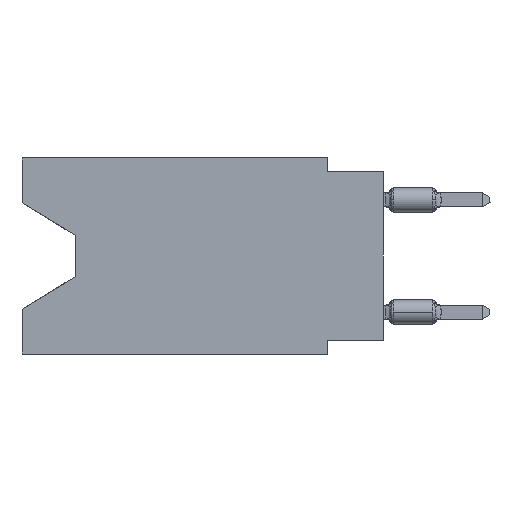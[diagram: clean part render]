
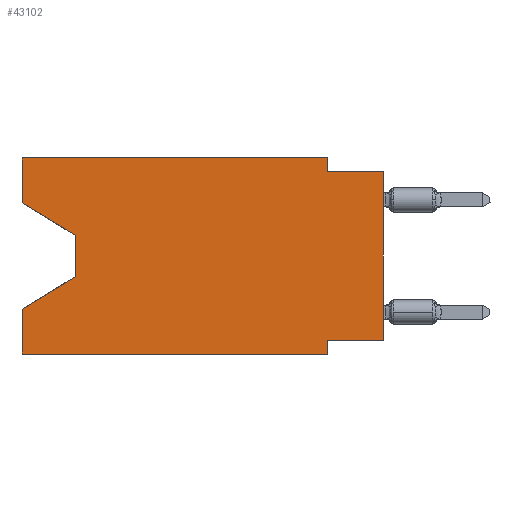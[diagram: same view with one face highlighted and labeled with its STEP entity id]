
A CAD part, left-side view. The second image highlights one B-rep face of the part: STEP entity #43102.
In plain terms, the highlighted planar face has unit normal (-1, 0, 0).
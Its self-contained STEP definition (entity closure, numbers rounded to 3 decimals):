
#617 = LINE ( 'NONE', #54633, #27802 ) ;
#1306 = VERTEX_POINT ( 'NONE', #27638 ) ;
#1836 = DIRECTION ( 'NONE',  ( 0., -1., 0. ) ) ;
#2307 = VERTEX_POINT ( 'NONE', #68463 ) ;
#2730 = EDGE_CURVE ( 'NONE', #19771, #59500, #4900, .T. ) ;
#3087 = DIRECTION ( 'NONE',  ( 0., 1., 0. ) ) ;
#3931 = DIRECTION ( 'NONE',  ( 0., -1., 0. ) ) ;
#4218 = ORIENTED_EDGE ( 'NONE', *, *, #52696, .F. ) ;
#4465 = LINE ( 'NONE', #56448, #4756 ) ;
#4756 = VECTOR ( 'NONE', #3087, 1000. ) ;
#4897 = VECTOR ( 'NONE', #27352, 1000. ) ;
#4900 = LINE ( 'NONE', #68368, #45089 ) ;
#5385 = CARTESIAN_POINT ( 'NONE',  ( 0., 16.383, 0. ) ) ;
#5423 = LINE ( 'NONE', #26704, #20906 ) ;
#5783 = EDGE_CURVE ( 'NONE', #59500, #37908, #5423, .T. ) ;
#5933 = VECTOR ( 'NONE', #34104, 1000. ) ;
#8051 = ORIENTED_EDGE ( 'NONE', *, *, #11867, .F. ) ;
#8557 = VECTOR ( 'NONE', #19544, 1000. ) ;
#9963 = DIRECTION ( 'NONE',  ( 0., 0.855, -0.519 ) ) ;
#11725 = ORIENTED_EDGE ( 'NONE', *, *, #42154, .T. ) ;
#11867 = EDGE_CURVE ( 'NONE', #49075, #37908, #66022, .T. ) ;
#11931 = CARTESIAN_POINT ( 'NONE',  ( 0., 2.54, -8.89 ) ) ;
#13270 = ORIENTED_EDGE ( 'NONE', *, *, #65249, .T. ) ;
#13945 = PLANE ( 'NONE',  #50484 ) ;
#14165 = VERTEX_POINT ( 'NONE', #53018 ) ;
#14279 = DIRECTION ( 'NONE',  ( 0., 0., -1. ) ) ;
#14666 = LINE ( 'NONE', #20944, #49072 ) ;
#15368 = LINE ( 'NONE', #58949, #54455 ) ;
#15716 = DIRECTION ( 'NONE',  ( 0., -1., 0. ) ) ;
#15976 = EDGE_CURVE ( 'NONE', #1306, #50974, #45350, .T. ) ;
#16616 = ORIENTED_EDGE ( 'NONE', *, *, #5783, .T. ) ;
#17039 = ORIENTED_EDGE ( 'NONE', *, *, #15976, .F. ) ;
#19544 = DIRECTION ( 'NONE',  ( 0., 0., -1. ) ) ;
#19771 = VERTEX_POINT ( 'NONE', #51970 ) ;
#19848 = EDGE_CURVE ( 'NONE', #2307, #37178, #14666, .T. ) ;
#20010 = CARTESIAN_POINT ( 'NONE',  ( 0., 16.383, 0. ) ) ;
#20029 = CARTESIAN_POINT ( 'NONE',  ( 0., 16.383, -2.038 ) ) ;
#20906 = VECTOR ( 'NONE', #9963, 1000. ) ;
#20944 = CARTESIAN_POINT ( 'NONE',  ( 0., 0., 0. ) ) ;
#21397 = EDGE_CURVE ( 'NONE', #14165, #37178, #51700, .T. ) ;
#23742 = CARTESIAN_POINT ( 'NONE',  ( 0., 2.54, -8.89 ) ) ;
#24390 = CARTESIAN_POINT ( 'NONE',  ( 0., 16.383, 0. ) ) ;
#26704 = CARTESIAN_POINT ( 'NONE',  ( 0., 13.97, -5.385 ) ) ;
#26950 = EDGE_CURVE ( 'NONE', #49923, #14165, #617, .T. ) ;
#27352 = DIRECTION ( 'NONE',  ( 0., 0., 1. ) ) ;
#27638 = CARTESIAN_POINT ( 'NONE',  ( 0., 2.54, -8.255 ) ) ;
#27802 = VECTOR ( 'NONE', #38603, 1000. ) ;
#28350 = CARTESIAN_POINT ( 'NONE',  ( 0., 16.383, -8.89 ) ) ;
#29972 = FACE_OUTER_BOUND ( 'NONE', #57995, .T. ) ;
#34005 = ORIENTED_EDGE ( 'NONE', *, *, #19848, .T. ) ;
#34104 = DIRECTION ( 'NONE',  ( 0., -0.855, -0.519 ) ) ;
#34168 = VERTEX_POINT ( 'NONE', #53078 ) ;
#34519 = DIRECTION ( 'NONE',  ( 1., 0., 0. ) ) ;
#34909 = CARTESIAN_POINT ( 'NONE',  ( 0., 2.54, 0. ) ) ;
#35396 = CARTESIAN_POINT ( 'NONE',  ( 0., 16.383, -8.89 ) ) ;
#36619 = CARTESIAN_POINT ( 'NONE',  ( 0., 13.97, -5.385 ) ) ;
#36625 = DIRECTION ( 'NONE',  ( 0., 0., -1. ) ) ;
#37178 = VERTEX_POINT ( 'NONE', #68458 ) ;
#37908 = VERTEX_POINT ( 'NONE', #45283 ) ;
#38603 = DIRECTION ( 'NONE',  ( 0., 0., -1. ) ) ;
#39521 = DIRECTION ( 'NONE',  ( 0., 0., 1. ) ) ;
#39584 = VERTEX_POINT ( 'NONE', #20010 ) ;
#41589 = CARTESIAN_POINT ( 'NONE',  ( 0., 0., -0.635 ) ) ;
#42009 = ORIENTED_EDGE ( 'NONE', *, *, #2730, .T. ) ;
#42154 = EDGE_CURVE ( 'NONE', #49075, #50974, #54835, .T. ) ;
#43102 = ADVANCED_FACE ( 'NONE', ( #29972 ), #13945, .F. ) ;
#43617 = EDGE_CURVE ( 'NONE', #34168, #39584, #53839, .T. ) ;
#43646 = VECTOR ( 'NONE', #39521, 1000. ) ;
#45089 = VECTOR ( 'NONE', #36625, 1000. ) ;
#45283 = CARTESIAN_POINT ( 'NONE',  ( 0., 16.383, -6.852 ) ) ;
#45350 = LINE ( 'NONE', #23742, #8557 ) ;
#45729 = ORIENTED_EDGE ( 'NONE', *, *, #66493, .F. ) ;
#48382 = CARTESIAN_POINT ( 'NONE',  ( 0., 16.383, 0. ) ) ;
#49072 = VECTOR ( 'NONE', #58599, 1000. ) ;
#49075 = VERTEX_POINT ( 'NONE', #35396 ) ;
#49923 = VERTEX_POINT ( 'NONE', #34909 ) ;
#50484 = AXIS2_PLACEMENT_3D ( 'NONE', #24390, #34519, #14279 ) ;
#50974 = VERTEX_POINT ( 'NONE', #11931 ) ;
#51513 = VECTOR ( 'NONE', #1836, 1000. ) ;
#51700 = LINE ( 'NONE', #41589, #63679 ) ;
#51970 = CARTESIAN_POINT ( 'NONE',  ( 0., 13.97, -3.505 ) ) ;
#52696 = EDGE_CURVE ( 'NONE', #2307, #1306, #4465, .T. ) ;
#53018 = CARTESIAN_POINT ( 'NONE',  ( 0., 2.54, -0.635 ) ) ;
#53078 = CARTESIAN_POINT ( 'NONE',  ( 0., 16.383, -2.038 ) ) ;
#53839 = LINE ( 'NONE', #5385, #4897 ) ;
#54455 = VECTOR ( 'NONE', #15716, 1000. ) ;
#54633 = CARTESIAN_POINT ( 'NONE',  ( 0., 2.54, 0. ) ) ;
#54835 = LINE ( 'NONE', #28350, #51513 ) ;
#56448 = CARTESIAN_POINT ( 'NONE',  ( 0., 0., -8.255 ) ) ;
#56814 = ORIENTED_EDGE ( 'NONE', *, *, #21397, .F. ) ;
#57431 = ORIENTED_EDGE ( 'NONE', *, *, #43617, .F. ) ;
#57995 = EDGE_LOOP ( 'NONE', ( #13270, #42009, #16616, #8051, #11725, #17039, #4218, #34005, #56814, #58733, #45729, #57431 ) ) ;
#58599 = DIRECTION ( 'NONE',  ( 0., 0., 1. ) ) ;
#58733 = ORIENTED_EDGE ( 'NONE', *, *, #26950, .F. ) ;
#58949 = CARTESIAN_POINT ( 'NONE',  ( 0., 16.383, 0. ) ) ;
#59500 = VERTEX_POINT ( 'NONE', #36619 ) ;
#63679 = VECTOR ( 'NONE', #3931, 1000. ) ;
#65249 = EDGE_CURVE ( 'NONE', #34168, #19771, #67800, .T. ) ;
#66022 = LINE ( 'NONE', #48382, #43646 ) ;
#66493 = EDGE_CURVE ( 'NONE', #39584, #49923, #15368, .T. ) ;
#67800 = LINE ( 'NONE', #20029, #5933 ) ;
#68368 = CARTESIAN_POINT ( 'NONE',  ( 0., 13.97, -3.505 ) ) ;
#68458 = CARTESIAN_POINT ( 'NONE',  ( 0., 0., -0.635 ) ) ;
#68463 = CARTESIAN_POINT ( 'NONE',  ( 0., 0., -8.255 ) ) ;
